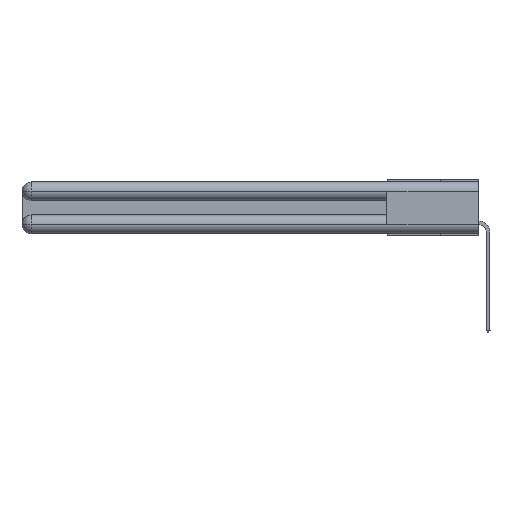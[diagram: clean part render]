
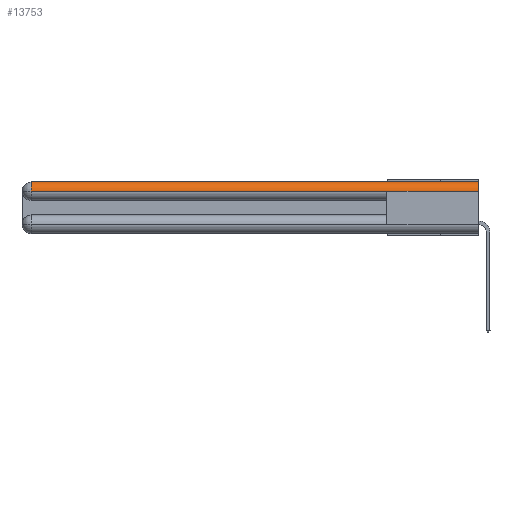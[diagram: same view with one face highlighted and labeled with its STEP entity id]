
A CAD part, left-side view. The second image highlights one B-rep face of the part: STEP entity #13753.
In plain terms, the highlighted cylindrical face has radius 1.562 mm (diameter 3.124 mm), a partial arc.
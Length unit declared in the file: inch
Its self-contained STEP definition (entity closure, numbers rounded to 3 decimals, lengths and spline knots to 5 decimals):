
#1799 = CARTESIAN_POINT ( 'NONE',  ( 0.0615, 0., 0. ) ) ;
#1928 = DIRECTION ( 'NONE',  ( 0., 0., 1. ) ) ;
#3483 = FACE_OUTER_BOUND ( 'NONE', #6913, .T. ) ;
#3762 = VERTEX_POINT ( 'NONE', #23369 ) ;
#4598 = CARTESIAN_POINT ( 'NONE',  ( 0., 0., -0.0615 ) ) ;
#4690 = VERTEX_POINT ( 'NONE', #14146 ) ;
#6913 = EDGE_LOOP ( 'NONE', ( #29284, #12222, #23878, #16884, #9159 ) ) ;
#9159 = ORIENTED_EDGE ( 'NONE', *, *, #21183, .F. ) ;
#10035 = CARTESIAN_POINT ( 'NONE',  ( 0.0615, 2.94, -0.0615 ) ) ;
#10578 = DIRECTION ( 'NONE',  ( 1., 0., 0. ) ) ;
#11550 = DIRECTION ( 'NONE',  ( 0., 1., 0. ) ) ;
#12222 = ORIENTED_EDGE ( 'NONE', *, *, #29898, .T. ) ;
#13753 = ADVANCED_FACE ( 'NONE', ( #3483 ), #23286, .T. ) ;
#14017 = CARTESIAN_POINT ( 'NONE',  ( 0.0615, 0., -0.0615 ) ) ;
#14146 = CARTESIAN_POINT ( 'NONE',  ( 0.0615, 2.94, 0. ) ) ;
#16241 = AXIS2_PLACEMENT_3D ( 'NONE', #25026, #27865, #10578 ) ;
#16471 = DIRECTION ( 'NONE',  ( 0., 1., 0. ) ) ;
#16884 = ORIENTED_EDGE ( 'NONE', *, *, #18912, .F. ) ;
#17671 = DIRECTION ( 'NONE',  ( 0., 0., 1. ) ) ;
#18912 = EDGE_CURVE ( 'NONE', #24772, #3762, #31380, .T. ) ;
#20806 = CARTESIAN_POINT ( 'NONE',  ( 0.0615, 0., 0. ) ) ;
#21183 = EDGE_CURVE ( 'NONE', #25188, #24772, #24949, .T. ) ;
#21571 = LINE ( 'NONE', #1799, #31052 ) ;
#22302 = CIRCLE ( 'NONE', #23936, 0.0615 ) ;
#22674 = VERTEX_POINT ( 'NONE', #24141 ) ;
#23286 = CYLINDRICAL_SURFACE ( 'NONE', #23333, 0.0615 ) ;
#23333 = AXIS2_PLACEMENT_3D ( 'NONE', #14017, #16471, #1928 ) ;
#23369 = CARTESIAN_POINT ( 'NONE',  ( 0., 0.6, -0.0615 ) ) ;
#23878 = ORIENTED_EDGE ( 'NONE', *, *, #28389, .T. ) ;
#23936 = AXIS2_PLACEMENT_3D ( 'NONE', #10035, #29651, #17671 ) ;
#24141 = CARTESIAN_POINT ( 'NONE',  ( 0., 2.94, -0.0615 ) ) ;
#24772 = VERTEX_POINT ( 'NONE', #4598 ) ;
#24949 = CIRCLE ( 'NONE', #16241, 0.0615 ) ;
#25026 = CARTESIAN_POINT ( 'NONE',  ( 0.0615, 0., -0.0615 ) ) ;
#25188 = VERTEX_POINT ( 'NONE', #20806 ) ;
#26100 = CARTESIAN_POINT ( 'NONE',  ( 0., 3., -0.0615 ) ) ;
#27252 = VECTOR ( 'NONE', #29871, 39.37008 ) ;
#27865 = DIRECTION ( 'NONE',  ( 0., -1., 0. ) ) ;
#28354 = DIRECTION ( 'NONE',  ( 0., -1., 0. ) ) ;
#28389 = EDGE_CURVE ( 'NONE', #22674, #3762, #30941, .T. ) ;
#29284 = ORIENTED_EDGE ( 'NONE', *, *, #29619, .F. ) ;
#29619 = EDGE_CURVE ( 'NONE', #4690, #25188, #21571, .T. ) ;
#29651 = DIRECTION ( 'NONE',  ( 0., -1., 0. ) ) ;
#29871 = DIRECTION ( 'NONE',  ( 0., -1., 0. ) ) ;
#29898 = EDGE_CURVE ( 'NONE', #4690, #22674, #22302, .T. ) ;
#30245 = VECTOR ( 'NONE', #11550, 39.37008 ) ;
#30284 = CARTESIAN_POINT ( 'NONE',  ( 0., 3., -0.0615 ) ) ;
#30941 = LINE ( 'NONE', #30284, #27252 ) ;
#31052 = VECTOR ( 'NONE', #28354, 39.37008 ) ;
#31380 = LINE ( 'NONE', #26100, #30245 ) ;
